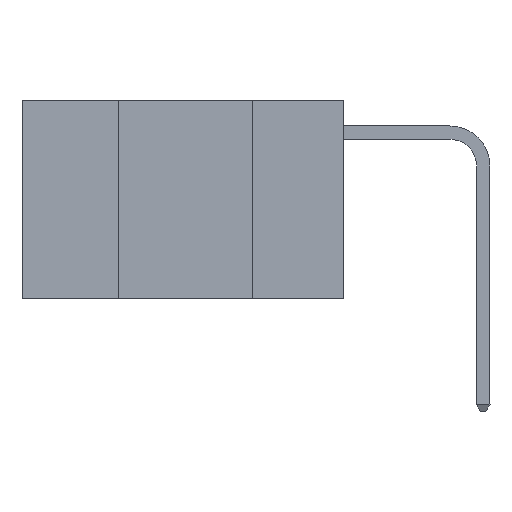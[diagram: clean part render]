
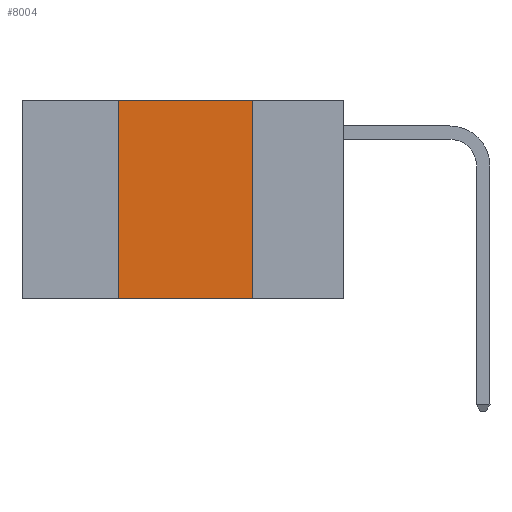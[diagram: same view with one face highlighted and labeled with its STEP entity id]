
A CAD part, left-side view. The second image highlights one B-rep face of the part: STEP entity #8004.
In plain terms, the highlighted planar face has unit normal (-1, 0, 0).
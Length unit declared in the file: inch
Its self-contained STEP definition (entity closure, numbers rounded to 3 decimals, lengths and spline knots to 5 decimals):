
#55 = DIRECTION ( 'NONE',  ( 0., 0., -1. ) ) ;
#770 = LINE ( 'NONE', #10473, #6498 ) ;
#2092 = PLANE ( 'NONE',  #12986 ) ;
#2305 = CARTESIAN_POINT ( 'NONE',  ( 0., 0.17, 0. ) ) ;
#2405 = CARTESIAN_POINT ( 'NONE',  ( 0., 0.42, 0. ) ) ;
#2491 = CARTESIAN_POINT ( 'NONE',  ( 0., 0.42, 0. ) ) ;
#3897 = CARTESIAN_POINT ( 'NONE',  ( 0., 0.17, 0. ) ) ;
#4162 = ORIENTED_EDGE ( 'NONE', *, *, #9684, .F. ) ;
#4163 = LINE ( 'NONE', #2491, #12836 ) ;
#4375 = DIRECTION ( 'NONE',  ( 1., 0., 0. ) ) ;
#4758 = DIRECTION ( 'NONE',  ( 0., -1., 0. ) ) ;
#5297 = LINE ( 'NONE', #2305, #10663 ) ;
#5601 = ORIENTED_EDGE ( 'NONE', *, *, #11889, .F. ) ;
#5681 = VERTEX_POINT ( 'NONE', #2405 ) ;
#5823 = FACE_OUTER_BOUND ( 'NONE', #7252, .T. ) ;
#6498 = VECTOR ( 'NONE', #4758, 39.37008 ) ;
#7027 = DIRECTION ( 'NONE',  ( 0., 0., 1. ) ) ;
#7252 = EDGE_LOOP ( 'NONE', ( #4162, #10945, #5601, #12650 ) ) ;
#7452 = EDGE_CURVE ( 'NONE', #5681, #11398, #7625, .T. ) ;
#7625 = LINE ( 'NONE', #9131, #10314 ) ;
#8004 = ADVANCED_FACE ( 'NONE', ( #5823 ), #2092, .F. ) ;
#9131 = CARTESIAN_POINT ( 'NONE',  ( 0., 0.6, 0. ) ) ;
#9418 = CARTESIAN_POINT ( 'NONE',  ( 0., 0.42, -0.37 ) ) ;
#9684 = EDGE_CURVE ( 'NONE', #11398, #12822, #5297, .T. ) ;
#10067 = CARTESIAN_POINT ( 'NONE',  ( 0., 0.17, -0.37 ) ) ;
#10296 = DIRECTION ( 'NONE',  ( 0., -1., 0. ) ) ;
#10314 = VECTOR ( 'NONE', #10296, 39.37008 ) ;
#10473 = CARTESIAN_POINT ( 'NONE',  ( 0., 0.6, -0.37 ) ) ;
#10663 = VECTOR ( 'NONE', #55, 39.37008 ) ;
#10945 = ORIENTED_EDGE ( 'NONE', *, *, #7452, .F. ) ;
#11201 = CARTESIAN_POINT ( 'NONE',  ( 0., 0.6, 0. ) ) ;
#11398 = VERTEX_POINT ( 'NONE', #3897 ) ;
#11889 = EDGE_CURVE ( 'NONE', #14225, #5681, #4163, .T. ) ;
#11914 = EDGE_CURVE ( 'NONE', #14225, #12822, #770, .T. ) ;
#12320 = DIRECTION ( 'NONE',  ( 0., 0., -1. ) ) ;
#12650 = ORIENTED_EDGE ( 'NONE', *, *, #11914, .T. ) ;
#12822 = VERTEX_POINT ( 'NONE', #10067 ) ;
#12836 = VECTOR ( 'NONE', #7027, 39.37008 ) ;
#12986 = AXIS2_PLACEMENT_3D ( 'NONE', #11201, #4375, #12320 ) ;
#14225 = VERTEX_POINT ( 'NONE', #9418 ) ;
